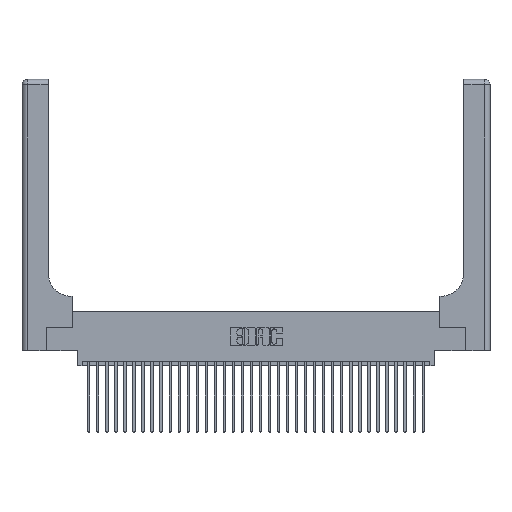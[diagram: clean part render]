
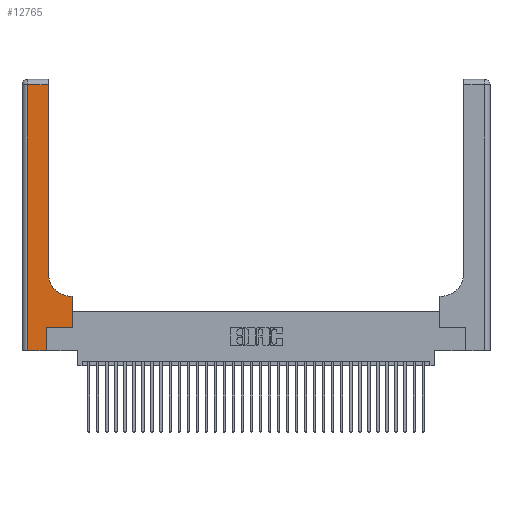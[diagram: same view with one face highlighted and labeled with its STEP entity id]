
A CAD part, top view. The second image highlights one B-rep face of the part: STEP entity #12765.
In plain terms, the highlighted planar face has unit normal (0, 0, 1).
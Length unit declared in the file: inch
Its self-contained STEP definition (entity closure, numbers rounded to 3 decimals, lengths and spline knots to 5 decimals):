
#330 = VECTOR ( 'NONE', #31453, 39.37008 ) ;
#721 = VERTEX_POINT ( 'NONE', #7499 ) ;
#1000 = EDGE_CURVE ( 'NONE', #9474, #17028, #14754, .T. ) ;
#1176 = DIRECTION ( 'NONE',  ( 0., 1., 0. ) ) ;
#1189 = VECTOR ( 'NONE', #26313, 39.37008 ) ;
#1233 = VERTEX_POINT ( 'NONE', #11856 ) ;
#1332 = ORIENTED_EDGE ( 'NONE', *, *, #2126, .T. ) ;
#1436 = EDGE_CURVE ( 'NONE', #1233, #33189, #14317, .T. ) ;
#1756 = VECTOR ( 'NONE', #19671, 39.37008 ) ;
#2126 = EDGE_CURVE ( 'NONE', #721, #12949, #5624, .T. ) ;
#2556 = ORIENTED_EDGE ( 'NONE', *, *, #1436, .T. ) ;
#2883 = DIRECTION ( 'NONE',  ( 0., 0., -1. ) ) ;
#3505 = EDGE_CURVE ( 'NONE', #16527, #9474, #20164, .T. ) ;
#4046 = CARTESIAN_POINT ( 'NONE',  ( 0.5585, 0.25, 0.37 ) ) ;
#4139 = AXIS2_PLACEMENT_3D ( 'NONE', #19071, #21864, #24630 ) ;
#4211 = ORIENTED_EDGE ( 'NONE', *, *, #22654, .T. ) ;
#5059 = VECTOR ( 'NONE', #22378, 39.37008 ) ;
#5365 = ORIENTED_EDGE ( 'NONE', *, *, #6501, .T. ) ;
#5587 = EDGE_LOOP ( 'NONE', ( #2556, #26950, #1332, #4211, #5365, #25261, #28003, #28800, #18588 ) ) ;
#5624 = LINE ( 'NONE', #25100, #1756 ) ;
#6392 = LINE ( 'NONE', #7909, #330 ) ;
#6501 = EDGE_CURVE ( 'NONE', #17253, #16527, #6392, .T. ) ;
#6800 = LINE ( 'NONE', #9949, #1189 ) ;
#7499 = CARTESIAN_POINT ( 'NONE',  ( 0.06, 2.94, 0.37 ) ) ;
#7909 = CARTESIAN_POINT ( 'NONE',  ( 0.269, 0., 0.37 ) ) ;
#7994 = VERTEX_POINT ( 'NONE', #20590 ) ;
#9474 = VERTEX_POINT ( 'NONE', #16374 ) ;
#9949 = CARTESIAN_POINT ( 'NONE',  ( 0., 2.94, 0.37 ) ) ;
#10714 = FACE_OUTER_BOUND ( 'NONE', #5587, .T. ) ;
#10804 = CARTESIAN_POINT ( 'NONE',  ( 0., 0., 0.37 ) ) ;
#10821 = DIRECTION ( 'NONE',  ( -1., 0., 0. ) ) ;
#11856 = CARTESIAN_POINT ( 'NONE',  ( 0.2915, 0.85, 0.37 ) ) ;
#12182 = CARTESIAN_POINT ( 'NONE',  ( 0.2915, 2.94, 0.37 ) ) ;
#12765 = ADVANCED_FACE ( 'NONE', ( #10714 ), #29974, .F. ) ;
#12949 = VERTEX_POINT ( 'NONE', #32173 ) ;
#13478 = VECTOR ( 'NONE', #1176, 39.37008 ) ;
#13612 = EDGE_CURVE ( 'NONE', #7994, #1233, #24277, .T. ) ;
#14317 = LINE ( 'NONE', #17786, #13478 ) ;
#14353 = CARTESIAN_POINT ( 'NONE',  ( 0.269, 0.25, 0.37 ) ) ;
#14754 = LINE ( 'NONE', #4046, #22087 ) ;
#15773 = CARTESIAN_POINT ( 'NONE',  ( 0.269, 0.25, 0.37 ) ) ;
#16374 = CARTESIAN_POINT ( 'NONE',  ( 0.5585, 0.25, 0.37 ) ) ;
#16527 = VERTEX_POINT ( 'NONE', #15773 ) ;
#16743 = VECTOR ( 'NONE', #33670, 39.37008 ) ;
#16932 = CARTESIAN_POINT ( 'NONE',  ( 0.2915, 0.6, 0.37 ) ) ;
#17028 = VERTEX_POINT ( 'NONE', #22337 ) ;
#17253 = VERTEX_POINT ( 'NONE', #18079 ) ;
#17786 = CARTESIAN_POINT ( 'NONE',  ( 0.2915, 3., 0.37 ) ) ;
#18079 = CARTESIAN_POINT ( 'NONE',  ( 0.269, 0., 0.37 ) ) ;
#18588 = ORIENTED_EDGE ( 'NONE', *, *, #13612, .T. ) ;
#19071 = CARTESIAN_POINT ( 'NONE',  ( 0.5415, 0.85, 0.37 ) ) ;
#19671 = DIRECTION ( 'NONE',  ( 0., -1., 0. ) ) ;
#20164 = LINE ( 'NONE', #14353, #23631 ) ;
#20590 = CARTESIAN_POINT ( 'NONE',  ( 0.5415, 0.6, 0.37 ) ) ;
#21796 = CARTESIAN_POINT ( 'NONE',  ( 0., 3., 0.37 ) ) ;
#21864 = DIRECTION ( 'NONE',  ( 0., 0., -1. ) ) ;
#22087 = VECTOR ( 'NONE', #23536, 39.37008 ) ;
#22337 = CARTESIAN_POINT ( 'NONE',  ( 0.5585, 0.6, 0.37 ) ) ;
#22378 = DIRECTION ( 'NONE',  ( -1., 0., 0. ) ) ;
#22654 = EDGE_CURVE ( 'NONE', #12949, #17253, #28797, .T. ) ;
#23536 = DIRECTION ( 'NONE',  ( 0., 1., 0. ) ) ;
#23631 = VECTOR ( 'NONE', #28163, 39.37008 ) ;
#24277 = CIRCLE ( 'NONE', #4139, 0.25 ) ;
#24630 = DIRECTION ( 'NONE',  ( 1., 0., 0. ) ) ;
#25100 = CARTESIAN_POINT ( 'NONE',  ( 0.06, 3., 0.37 ) ) ;
#25261 = ORIENTED_EDGE ( 'NONE', *, *, #3505, .T. ) ;
#26313 = DIRECTION ( 'NONE',  ( -1., 0., 0. ) ) ;
#26452 = EDGE_CURVE ( 'NONE', #17028, #7994, #27849, .T. ) ;
#26950 = ORIENTED_EDGE ( 'NONE', *, *, #33918, .T. ) ;
#27433 = AXIS2_PLACEMENT_3D ( 'NONE', #21796, #2883, #10821 ) ;
#27849 = LINE ( 'NONE', #16932, #5059 ) ;
#28003 = ORIENTED_EDGE ( 'NONE', *, *, #1000, .T. ) ;
#28163 = DIRECTION ( 'NONE',  ( 1., 0., 0. ) ) ;
#28797 = LINE ( 'NONE', #10804, #16743 ) ;
#28800 = ORIENTED_EDGE ( 'NONE', *, *, #26452, .T. ) ;
#29974 = PLANE ( 'NONE',  #27433 ) ;
#31453 = DIRECTION ( 'NONE',  ( 0., 1., 0. ) ) ;
#32173 = CARTESIAN_POINT ( 'NONE',  ( 0.06, 0., 0.37 ) ) ;
#33189 = VERTEX_POINT ( 'NONE', #12182 ) ;
#33670 = DIRECTION ( 'NONE',  ( 1., 0., 0. ) ) ;
#33918 = EDGE_CURVE ( 'NONE', #33189, #721, #6800, .T. ) ;
